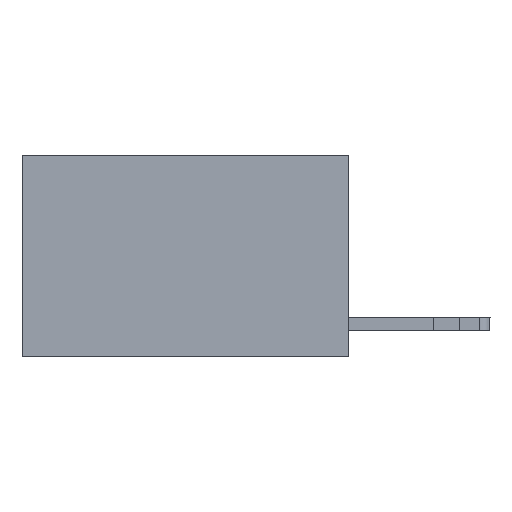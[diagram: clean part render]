
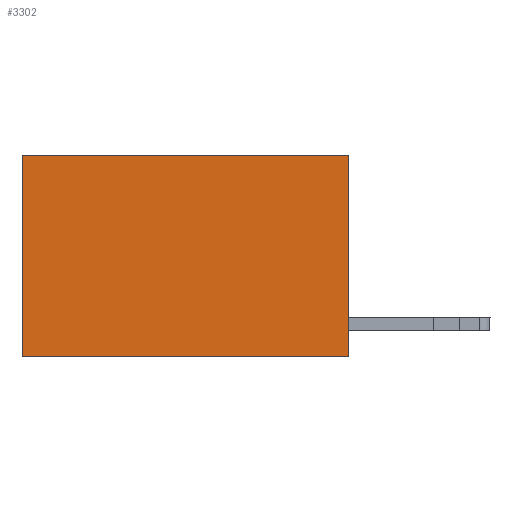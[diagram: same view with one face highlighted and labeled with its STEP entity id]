
A CAD part, left-side view. The second image highlights one B-rep face of the part: STEP entity #3302.
In plain terms, the highlighted planar face has unit normal (-1, 0, 0).
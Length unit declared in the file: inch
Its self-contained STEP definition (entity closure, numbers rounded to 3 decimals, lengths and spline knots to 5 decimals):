
#361 = DIRECTION ( 'NONE',  ( 0., 1., 0. ) ) ;
#418 = LINE ( 'NONE', #10885, #7916 ) ;
#431 = CARTESIAN_POINT ( 'NONE',  ( 0.2625, 0., -0.37 ) ) ;
#475 = VECTOR ( 'NONE', #19064, 39.37008 ) ;
#482 = LINE ( 'NONE', #18293, #15925 ) ;
#521 = DIRECTION ( 'NONE',  ( 0., 1., 0. ) ) ;
#1441 = CARTESIAN_POINT ( 'NONE',  ( 0.2625, 0., 0. ) ) ;
#2729 = CARTESIAN_POINT ( 'NONE',  ( 0.2625, 0., 0. ) ) ;
#3301 = VERTEX_POINT ( 'NONE', #18184 ) ;
#3302 = ADVANCED_FACE ( 'NONE', ( #4797 ), #15397, .F. ) ;
#4209 = LINE ( 'NONE', #9332, #7715 ) ;
#4797 = FACE_OUTER_BOUND ( 'NONE', #8611, .T. ) ;
#4831 = ORIENTED_EDGE ( 'NONE', *, *, #6873, .T. ) ;
#6227 = EDGE_CURVE ( 'NONE', #15795, #3301, #4209, .T. ) ;
#6478 = DIRECTION ( 'NONE',  ( 0., 0., -1. ) ) ;
#6509 = ORIENTED_EDGE ( 'NONE', *, *, #6227, .T. ) ;
#6873 = EDGE_CURVE ( 'NONE', #3301, #10493, #418, .T. ) ;
#7715 = VECTOR ( 'NONE', #521, 39.37008 ) ;
#7916 = VECTOR ( 'NONE', #12421, 39.37008 ) ;
#8611 = EDGE_LOOP ( 'NONE', ( #4831, #18144, #14123, #6509 ) ) ;
#9332 = CARTESIAN_POINT ( 'NONE',  ( 0.2625, 0., 0. ) ) ;
#9916 = DIRECTION ( 'NONE',  ( 1., 0., 0. ) ) ;
#10493 = VERTEX_POINT ( 'NONE', #13675 ) ;
#10567 = EDGE_CURVE ( 'NONE', #19188, #10493, #482, .T. ) ;
#10885 = CARTESIAN_POINT ( 'NONE',  ( 0.2625, 0.6, 0. ) ) ;
#11536 = CARTESIAN_POINT ( 'NONE',  ( 0.2625, 0., 0. ) ) ;
#12421 = DIRECTION ( 'NONE',  ( 0., 0., -1. ) ) ;
#12435 = LINE ( 'NONE', #11536, #475 ) ;
#13675 = CARTESIAN_POINT ( 'NONE',  ( 0.2625, 0.6, -0.37 ) ) ;
#14123 = ORIENTED_EDGE ( 'NONE', *, *, #15636, .F. ) ;
#15397 = PLANE ( 'NONE',  #18081 ) ;
#15636 = EDGE_CURVE ( 'NONE', #15795, #19188, #12435, .T. ) ;
#15795 = VERTEX_POINT ( 'NONE', #1441 ) ;
#15925 = VECTOR ( 'NONE', #361, 39.37008 ) ;
#18081 = AXIS2_PLACEMENT_3D ( 'NONE', #2729, #9916, #6478 ) ;
#18144 = ORIENTED_EDGE ( 'NONE', *, *, #10567, .F. ) ;
#18184 = CARTESIAN_POINT ( 'NONE',  ( 0.2625, 0.6, 0. ) ) ;
#18293 = CARTESIAN_POINT ( 'NONE',  ( 0.2625, 0., -0.37 ) ) ;
#19064 = DIRECTION ( 'NONE',  ( 0., 0., -1. ) ) ;
#19188 = VERTEX_POINT ( 'NONE', #431 ) ;
